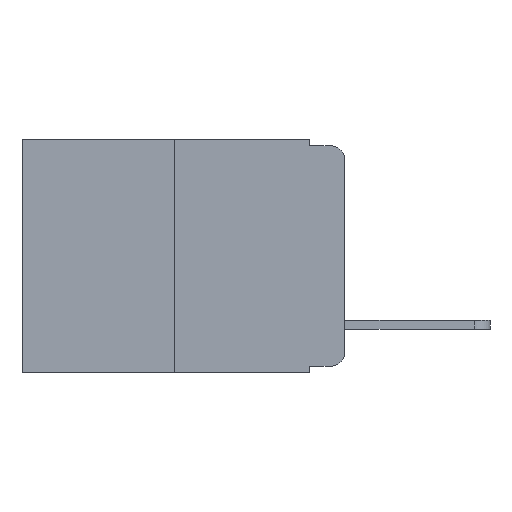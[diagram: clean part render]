
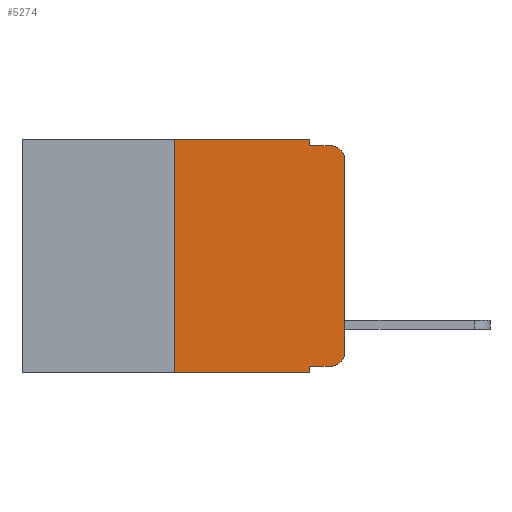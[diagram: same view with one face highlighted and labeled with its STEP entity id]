
A CAD part, left-side view. The second image highlights one B-rep face of the part: STEP entity #5274.
In plain terms, the highlighted planar face has unit normal (-1, 0, 0).
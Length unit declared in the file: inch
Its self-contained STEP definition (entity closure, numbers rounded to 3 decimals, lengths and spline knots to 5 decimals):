
#7 = AXIS2_PLACEMENT_3D ( 'NONE', #2381, #2459, #2448 ) ;
#220 = AXIS2_PLACEMENT_3D ( 'NONE', #10631, #11245, #11193 ) ;
#249 = VERTEX_POINT ( 'NONE', #3070 ) ;
#795 = LINE ( 'NONE', #10554, #10342 ) ;
#1000 = VECTOR ( 'NONE', #3043, 39.37008 ) ;
#1420 = VECTOR ( 'NONE', #4244, 39.37008 ) ;
#1459 = VERTEX_POINT ( 'NONE', #5754 ) ;
#1577 = DIRECTION ( 'NONE',  ( -1., 0., 0. ) ) ;
#1600 = CARTESIAN_POINT ( 'NONE',  ( 0., 0.02, -0.313 ) ) ;
#1997 = VERTEX_POINT ( 'NONE', #8792 ) ;
#2023 = VERTEX_POINT ( 'NONE', #5656 ) ;
#2381 = CARTESIAN_POINT ( 'NONE',  ( 0., 0.02, -0.03 ) ) ;
#2448 = DIRECTION ( 'NONE',  ( 0., 0., -1. ) ) ;
#2459 = DIRECTION ( 'NONE',  ( -1., 0., 0. ) ) ;
#2477 = VECTOR ( 'NONE', #9912, 39.37008 ) ;
#2851 = VERTEX_POINT ( 'NONE', #9954 ) ;
#3043 = DIRECTION ( 'NONE',  ( 0., 0., -1. ) ) ;
#3070 = CARTESIAN_POINT ( 'NONE',  ( 0., 0.051, -0.343 ) ) ;
#3106 = VERTEX_POINT ( 'NONE', #5263 ) ;
#3304 = VECTOR ( 'NONE', #9412, 39.37008 ) ;
#3461 = CIRCLE ( 'NONE', #4864, 0.02 ) ;
#3585 = VERTEX_POINT ( 'NONE', #7356 ) ;
#3906 = EDGE_CURVE ( 'NONE', #2851, #10674, #795, .T. ) ;
#4126 = FACE_OUTER_BOUND ( 'NONE', #4377, .T. ) ;
#4244 = DIRECTION ( 'NONE',  ( 0., 0., 1. ) ) ;
#4338 = CARTESIAN_POINT ( 'NONE',  ( 0., 0.25, 0. ) ) ;
#4377 = EDGE_LOOP ( 'NONE', ( #4489, #4507, #4629, #4656, #4677, #4712, #4741, #4843, #4917, #5016 ) ) ;
#4436 = VECTOR ( 'NONE', #9681, 39.37008 ) ;
#4489 = ORIENTED_EDGE ( 'NONE', *, *, #3906, .T. ) ;
#4507 = ORIENTED_EDGE ( 'NONE', *, *, #5068, .T. ) ;
#4629 = ORIENTED_EDGE ( 'NONE', *, *, #6130, .F. ) ;
#4650 = LINE ( 'NONE', #9803, #8326 ) ;
#4656 = ORIENTED_EDGE ( 'NONE', *, *, #5254, .F. ) ;
#4677 = ORIENTED_EDGE ( 'NONE', *, *, #10721, .F. ) ;
#4712 = ORIENTED_EDGE ( 'NONE', *, *, #7551, .F. ) ;
#4741 = ORIENTED_EDGE ( 'NONE', *, *, #11306, .T. ) ;
#4843 = ORIENTED_EDGE ( 'NONE', *, *, #5859, .F. ) ;
#4864 = AXIS2_PLACEMENT_3D ( 'NONE', #1600, #1577, #11496 ) ;
#4917 = ORIENTED_EDGE ( 'NONE', *, *, #5057, .T. ) ;
#5015 = CARTESIAN_POINT ( 'NONE',  ( 0., 0.25, 0. ) ) ;
#5016 = ORIENTED_EDGE ( 'NONE', *, *, #10898, .T. ) ;
#5057 = EDGE_CURVE ( 'NONE', #1459, #3106, #7745, .T. ) ;
#5068 = EDGE_CURVE ( 'NONE', #10674, #3585, #7500, .T. ) ;
#5254 = EDGE_CURVE ( 'NONE', #1997, #6172, #8674, .T. ) ;
#5263 = CARTESIAN_POINT ( 'NONE',  ( 0., 0.02, -0.333 ) ) ;
#5274 = ADVANCED_FACE ( 'NONE', ( #4126 ), #7896, .F. ) ;
#5298 = VECTOR ( 'NONE', #8321, 39.37008 ) ;
#5574 = CARTESIAN_POINT ( 'NONE',  ( 0., 0., -0.03 ) ) ;
#5656 = CARTESIAN_POINT ( 'NONE',  ( 0., 0.25, -0.343 ) ) ;
#5754 = CARTESIAN_POINT ( 'NONE',  ( 0., 0.051, -0.333 ) ) ;
#5859 = EDGE_CURVE ( 'NONE', #1459, #249, #9714, .T. ) ;
#6130 = EDGE_CURVE ( 'NONE', #6172, #3585, #9154, .T. ) ;
#6172 = VERTEX_POINT ( 'NONE', #10479 ) ;
#7313 = CARTESIAN_POINT ( 'NONE',  ( 0., 0.473, -0.343 ) ) ;
#7356 = CARTESIAN_POINT ( 'NONE',  ( 0., 0.02, -0.01 ) ) ;
#7438 = LINE ( 'NONE', #4338, #1420 ) ;
#7500 = CIRCLE ( 'NONE', #7, 0.02 ) ;
#7551 = EDGE_CURVE ( 'NONE', #2023, #8946, #7438, .T. ) ;
#7720 = CARTESIAN_POINT ( 'NONE',  ( 0., 0.051, -0.333 ) ) ;
#7745 = LINE ( 'NONE', #7720, #2477 ) ;
#7896 = PLANE ( 'NONE',  #220 ) ;
#8207 = LINE ( 'NONE', #7313, #3304 ) ;
#8279 = CARTESIAN_POINT ( 'NONE',  ( 0., 0.051, 0. ) ) ;
#8321 = DIRECTION ( 'NONE',  ( 0., 0., -1. ) ) ;
#8326 = VECTOR ( 'NONE', #9838, 39.37008 ) ;
#8674 = LINE ( 'NONE', #10865, #1000 ) ;
#8792 = CARTESIAN_POINT ( 'NONE',  ( 0., 0.051, 0. ) ) ;
#8946 = VERTEX_POINT ( 'NONE', #5015 ) ;
#9154 = LINE ( 'NONE', #9709, #4436 ) ;
#9412 = DIRECTION ( 'NONE',  ( 0., -1., 0. ) ) ;
#9681 = DIRECTION ( 'NONE',  ( 0., -1., 0. ) ) ;
#9709 = CARTESIAN_POINT ( 'NONE',  ( 0., 0.051, -0.01 ) ) ;
#9714 = LINE ( 'NONE', #8279, #5298 ) ;
#9803 = CARTESIAN_POINT ( 'NONE',  ( 0., 0.473, 0. ) ) ;
#9838 = DIRECTION ( 'NONE',  ( 0., -1., 0. ) ) ;
#9912 = DIRECTION ( 'NONE',  ( 0., -1., 0. ) ) ;
#9954 = CARTESIAN_POINT ( 'NONE',  ( 0., 0., -0.313 ) ) ;
#10342 = VECTOR ( 'NONE', #10533, 39.37008 ) ;
#10479 = CARTESIAN_POINT ( 'NONE',  ( 0., 0.051, -0.01 ) ) ;
#10533 = DIRECTION ( 'NONE',  ( 0., 0., 1. ) ) ;
#10554 = CARTESIAN_POINT ( 'NONE',  ( 0., 0., 0. ) ) ;
#10631 = CARTESIAN_POINT ( 'NONE',  ( 0., 0.473, 0. ) ) ;
#10674 = VERTEX_POINT ( 'NONE', #5574 ) ;
#10721 = EDGE_CURVE ( 'NONE', #8946, #1997, #4650, .T. ) ;
#10865 = CARTESIAN_POINT ( 'NONE',  ( 0., 0.051, 0. ) ) ;
#10898 = EDGE_CURVE ( 'NONE', #3106, #2851, #3461, .T. ) ;
#11193 = DIRECTION ( 'NONE',  ( 0., 0., -1. ) ) ;
#11245 = DIRECTION ( 'NONE',  ( 1., 0., 0. ) ) ;
#11306 = EDGE_CURVE ( 'NONE', #2023, #249, #8207, .T. ) ;
#11496 = DIRECTION ( 'NONE',  ( 0., 0., -1. ) ) ;
